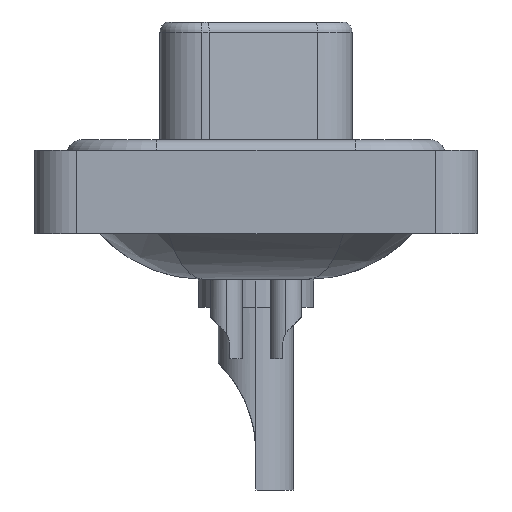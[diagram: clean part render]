
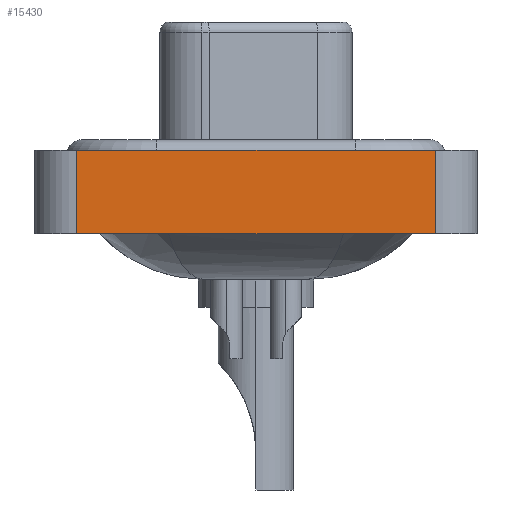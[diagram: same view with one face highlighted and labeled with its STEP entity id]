
A CAD part, left-side view. The second image highlights one B-rep face of the part: STEP entity #15430.
In plain terms, the highlighted planar face has unit normal (-1, 0, 0).
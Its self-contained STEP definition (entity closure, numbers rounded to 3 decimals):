
#1003 = LINE ( 'NONE', #9414, #11873 ) ;
#1558 = LINE ( 'NONE', #5722, #12937 ) ;
#2211 = DIRECTION ( 'NONE',  ( 0., 0., 1. ) ) ;
#2762 = VERTEX_POINT ( 'NONE', #18184 ) ;
#3483 = PLANE ( 'NONE',  #9248 ) ;
#4260 = DIRECTION ( 'NONE',  ( 0., -1., 0. ) ) ;
#4343 = ORIENTED_EDGE ( 'NONE', *, *, #5888, .F. ) ;
#5557 = CARTESIAN_POINT ( 'NONE',  ( -7.25, -8.55, -3.6 ) ) ;
#5722 = CARTESIAN_POINT ( 'NONE',  ( -7.25, -8.55, -3.6 ) ) ;
#5888 = EDGE_CURVE ( 'NONE', #12056, #16420, #1003, .T. ) ;
#6645 = VECTOR ( 'NONE', #2211, 1000. ) ;
#8955 = CARTESIAN_POINT ( 'NONE',  ( -7.25, 8.55, -3.6 ) ) ;
#9210 = DIRECTION ( 'NONE',  ( 0., 0., 1. ) ) ;
#9237 = LINE ( 'NONE', #9339, #6645 ) ;
#9248 = AXIS2_PLACEMENT_3D ( 'NONE', #16095, #17733, #9210 ) ;
#9339 = CARTESIAN_POINT ( 'NONE',  ( -7.25, 8.55, -3.6 ) ) ;
#9414 = CARTESIAN_POINT ( 'NONE',  ( -7.25, -8.55, 0.4 ) ) ;
#9747 = ORIENTED_EDGE ( 'NONE', *, *, #14758, .T. ) ;
#10087 = EDGE_CURVE ( 'NONE', #2762, #16420, #1558, .T. ) ;
#10293 = VERTEX_POINT ( 'NONE', #8955 ) ;
#10363 = EDGE_LOOP ( 'NONE', ( #13378, #4343, #17017, #9747 ) ) ;
#11873 = VECTOR ( 'NONE', #13890, 1000. ) ;
#12056 = VERTEX_POINT ( 'NONE', #16092 ) ;
#12166 = CARTESIAN_POINT ( 'NONE',  ( -7.25, -8.55, 0.4 ) ) ;
#12937 = VECTOR ( 'NONE', #15747, 1000. ) ;
#13320 = VECTOR ( 'NONE', #4260, 1000. ) ;
#13378 = ORIENTED_EDGE ( 'NONE', *, *, #10087, .T. ) ;
#13890 = DIRECTION ( 'NONE',  ( 0., -1., 0. ) ) ;
#14758 = EDGE_CURVE ( 'NONE', #10293, #2762, #15304, .T. ) ;
#14899 = FACE_OUTER_BOUND ( 'NONE', #10363, .T. ) ;
#15304 = LINE ( 'NONE', #5557, #13320 ) ;
#15430 = ADVANCED_FACE ( 'NONE', ( #14899 ), #3483, .T. ) ;
#15747 = DIRECTION ( 'NONE',  ( 0., 0., 1. ) ) ;
#16092 = CARTESIAN_POINT ( 'NONE',  ( -7.25, 8.55, 0.4 ) ) ;
#16095 = CARTESIAN_POINT ( 'NONE',  ( -7.25, -8.55, -3.6 ) ) ;
#16311 = EDGE_CURVE ( 'NONE', #10293, #12056, #9237, .T. ) ;
#16420 = VERTEX_POINT ( 'NONE', #12166 ) ;
#17017 = ORIENTED_EDGE ( 'NONE', *, *, #16311, .F. ) ;
#17733 = DIRECTION ( 'NONE',  ( -1., 0., 0. ) ) ;
#18184 = CARTESIAN_POINT ( 'NONE',  ( -7.25, -8.55, -3.6 ) ) ;
